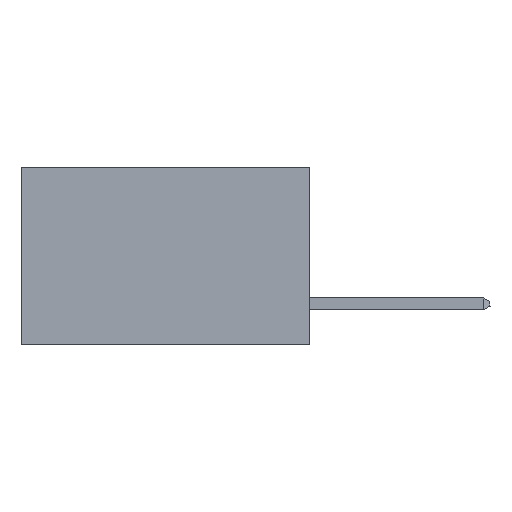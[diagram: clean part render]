
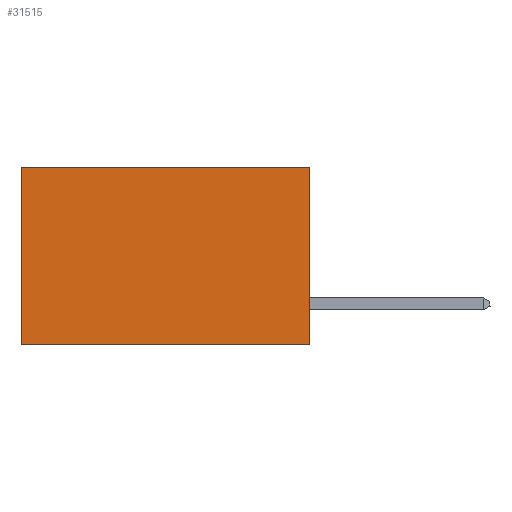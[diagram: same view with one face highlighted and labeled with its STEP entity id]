
A CAD part, left-side view. The second image highlights one B-rep face of the part: STEP entity #31515.
In plain terms, the highlighted planar face has unit normal (-1, 0, 0).
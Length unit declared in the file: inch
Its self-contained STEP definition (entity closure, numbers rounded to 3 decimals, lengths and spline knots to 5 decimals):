
#388 = VERTEX_POINT ( 'NONE', #12127 ) ;
#738 = ORIENTED_EDGE ( 'NONE', *, *, #15549, .T. ) ;
#746 = CARTESIAN_POINT ( 'NONE',  ( 0.2875, 0., -0.37 ) ) ;
#2610 = AXIS2_PLACEMENT_3D ( 'NONE', #7241, #32348, #17367 ) ;
#3406 = LINE ( 'NONE', #746, #23523 ) ;
#4313 = ORIENTED_EDGE ( 'NONE', *, *, #13595, .T. ) ;
#5431 = VECTOR ( 'NONE', #10244, 39.37008 ) ;
#6053 = VERTEX_POINT ( 'NONE', #12288 ) ;
#6426 = VECTOR ( 'NONE', #17234, 39.37008 ) ;
#7241 = CARTESIAN_POINT ( 'NONE',  ( 0.2875, 0., 0. ) ) ;
#7659 = CARTESIAN_POINT ( 'NONE',  ( 0.2875, 0., -0.37 ) ) ;
#7663 = CARTESIAN_POINT ( 'NONE',  ( 0.2875, 0., 0. ) ) ;
#8493 = DIRECTION ( 'NONE',  ( 0., 1., 0. ) ) ;
#10244 = DIRECTION ( 'NONE',  ( 0., 0., -1. ) ) ;
#12127 = CARTESIAN_POINT ( 'NONE',  ( 0.2875, 0.6, 0. ) ) ;
#12288 = CARTESIAN_POINT ( 'NONE',  ( 0.2875, 0., 0. ) ) ;
#13595 = EDGE_CURVE ( 'NONE', #388, #22458, #16792, .T. ) ;
#14568 = FACE_OUTER_BOUND ( 'NONE', #15204, .T. ) ;
#14762 = CARTESIAN_POINT ( 'NONE',  ( 0.2875, 0., 0. ) ) ;
#15027 = VERTEX_POINT ( 'NONE', #7659 ) ;
#15204 = EDGE_LOOP ( 'NONE', ( #4313, #17154, #22515, #738 ) ) ;
#15549 = EDGE_CURVE ( 'NONE', #6053, #388, #26501, .T. ) ;
#16792 = LINE ( 'NONE', #32262, #17549 ) ;
#17154 = ORIENTED_EDGE ( 'NONE', *, *, #20679, .F. ) ;
#17234 = DIRECTION ( 'NONE',  ( 0., 1., 0. ) ) ;
#17367 = DIRECTION ( 'NONE',  ( 0., 0., -1. ) ) ;
#17549 = VECTOR ( 'NONE', #19721, 39.37008 ) ;
#19475 = CARTESIAN_POINT ( 'NONE',  ( 0.2875, 0.6, -0.37 ) ) ;
#19721 = DIRECTION ( 'NONE',  ( 0., 0., -1. ) ) ;
#20679 = EDGE_CURVE ( 'NONE', #15027, #22458, #3406, .T. ) ;
#22458 = VERTEX_POINT ( 'NONE', #19475 ) ;
#22515 = ORIENTED_EDGE ( 'NONE', *, *, #31620, .F. ) ;
#23523 = VECTOR ( 'NONE', #8493, 39.37008 ) ;
#23996 = LINE ( 'NONE', #7663, #5431 ) ;
#26501 = LINE ( 'NONE', #14762, #6426 ) ;
#29892 = PLANE ( 'NONE',  #2610 ) ;
#31515 = ADVANCED_FACE ( 'NONE', ( #14568 ), #29892, .F. ) ;
#31620 = EDGE_CURVE ( 'NONE', #6053, #15027, #23996, .T. ) ;
#32262 = CARTESIAN_POINT ( 'NONE',  ( 0.2875, 0.6, 0. ) ) ;
#32348 = DIRECTION ( 'NONE',  ( 1., 0., 0. ) ) ;
